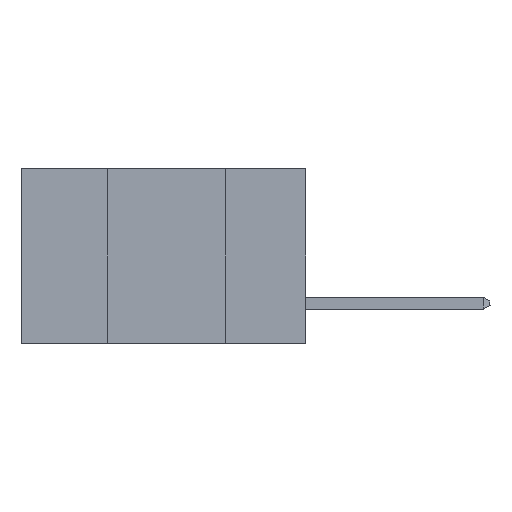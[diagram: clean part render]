
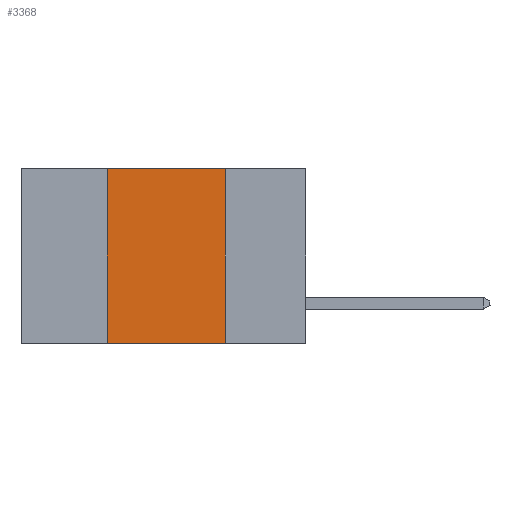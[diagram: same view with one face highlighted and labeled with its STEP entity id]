
A CAD part, left-side view. The second image highlights one B-rep face of the part: STEP entity #3368.
In plain terms, the highlighted planar face has unit normal (-1, 0, 0).
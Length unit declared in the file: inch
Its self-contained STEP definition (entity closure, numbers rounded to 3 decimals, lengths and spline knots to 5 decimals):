
#587 = EDGE_CURVE ( 'NONE', #15541, #4653, #4529, .T. ) ;
#1201 = AXIS2_PLACEMENT_3D ( 'NONE', #10204, #22501, #5063 ) ;
#1299 = EDGE_LOOP ( 'NONE', ( #13169, #6858, #19175, #19044 ) ) ;
#1533 = CARTESIAN_POINT ( 'NONE',  ( 0., 0.17, 0. ) ) ;
#1686 = LINE ( 'NONE', #7598, #9952 ) ;
#2015 = EDGE_CURVE ( 'NONE', #22071, #4653, #1686, .T. ) ;
#3357 = LINE ( 'NONE', #9449, #4191 ) ;
#3368 = ADVANCED_FACE ( 'NONE', ( #13731 ), #22346, .F. ) ;
#3438 = VERTEX_POINT ( 'NONE', #15968 ) ;
#3868 = CARTESIAN_POINT ( 'NONE',  ( 0., 0.17, 0. ) ) ;
#4191 = VECTOR ( 'NONE', #11366, 39.37008 ) ;
#4529 = LINE ( 'NONE', #1533, #22661 ) ;
#4653 = VERTEX_POINT ( 'NONE', #9009 ) ;
#5063 = DIRECTION ( 'NONE',  ( 0., 0., -1. ) ) ;
#5771 = VECTOR ( 'NONE', #14835, 39.37008 ) ;
#6058 = DIRECTION ( 'NONE',  ( 0., -1., 0. ) ) ;
#6858 = ORIENTED_EDGE ( 'NONE', *, *, #7408, .F. ) ;
#7408 = EDGE_CURVE ( 'NONE', #3438, #15541, #3357, .T. ) ;
#7598 = CARTESIAN_POINT ( 'NONE',  ( 0., 0.6, -0.37 ) ) ;
#7975 = LINE ( 'NONE', #21906, #5771 ) ;
#9009 = CARTESIAN_POINT ( 'NONE',  ( 0., 0.17, -0.37 ) ) ;
#9449 = CARTESIAN_POINT ( 'NONE',  ( 0., 0.6, 0. ) ) ;
#9952 = VECTOR ( 'NONE', #6058, 39.37008 ) ;
#10204 = CARTESIAN_POINT ( 'NONE',  ( 0., 0.6, 0. ) ) ;
#11366 = DIRECTION ( 'NONE',  ( 0., -1., 0. ) ) ;
#13169 = ORIENTED_EDGE ( 'NONE', *, *, #587, .F. ) ;
#13259 = EDGE_CURVE ( 'NONE', #22071, #3438, #7975, .T. ) ;
#13731 = FACE_OUTER_BOUND ( 'NONE', #1299, .T. ) ;
#14835 = DIRECTION ( 'NONE',  ( 0., 0., 1. ) ) ;
#15541 = VERTEX_POINT ( 'NONE', #3868 ) ;
#15968 = CARTESIAN_POINT ( 'NONE',  ( 0., 0.42, 0. ) ) ;
#16803 = CARTESIAN_POINT ( 'NONE',  ( 0., 0.42, -0.37 ) ) ;
#18066 = DIRECTION ( 'NONE',  ( 0., 0., -1. ) ) ;
#19044 = ORIENTED_EDGE ( 'NONE', *, *, #2015, .T. ) ;
#19175 = ORIENTED_EDGE ( 'NONE', *, *, #13259, .F. ) ;
#21906 = CARTESIAN_POINT ( 'NONE',  ( 0., 0.42, 0. ) ) ;
#22071 = VERTEX_POINT ( 'NONE', #16803 ) ;
#22346 = PLANE ( 'NONE',  #1201 ) ;
#22501 = DIRECTION ( 'NONE',  ( 1., 0., 0. ) ) ;
#22661 = VECTOR ( 'NONE', #18066, 39.37008 ) ;
